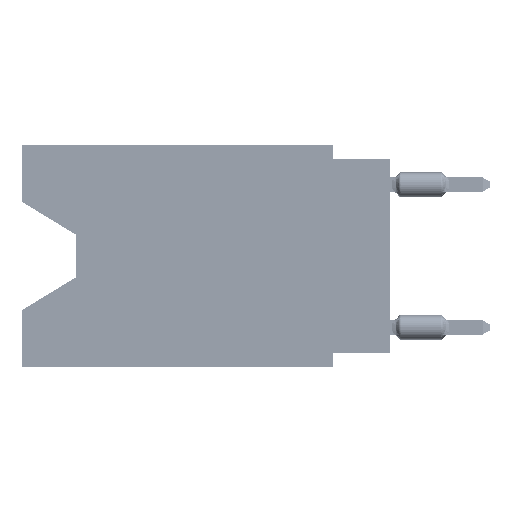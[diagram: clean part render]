
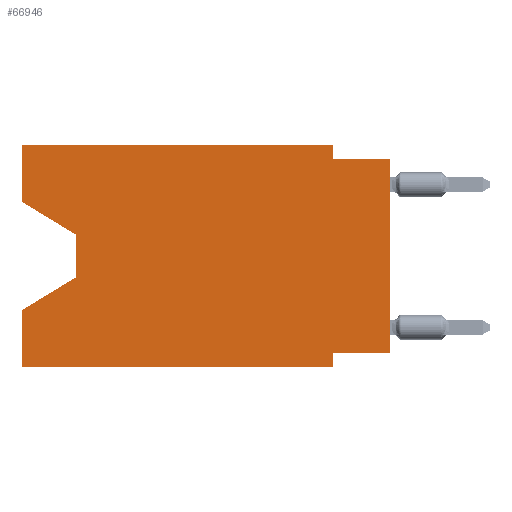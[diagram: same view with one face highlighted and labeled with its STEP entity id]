
A CAD part, left-side view. The second image highlights one B-rep face of the part: STEP entity #66946.
In plain terms, the highlighted planar face has unit normal (-1, 0, 0).
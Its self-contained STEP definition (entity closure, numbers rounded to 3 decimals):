
#549 = EDGE_CURVE ( 'NONE', #31729, #74322, #68696, .T. ) ;
#580 = DIRECTION ( 'NONE',  ( 0., 0., -1. ) ) ;
#655 = ORIENTED_EDGE ( 'NONE', *, *, #60571, .T. ) ;
#4515 = LINE ( 'NONE', #27219, #60084 ) ;
#5648 = EDGE_CURVE ( 'NONE', #44229, #64626, #75842, .T. ) ;
#5775 = CARTESIAN_POINT ( 'NONE',  ( 0., 13.97, -4.013 ) ) ;
#6532 = CARTESIAN_POINT ( 'NONE',  ( 0., 13.97, -4.013 ) ) ;
#7462 = DIRECTION ( 'NONE',  ( 0., -1., 0. ) ) ;
#8354 = CARTESIAN_POINT ( 'NONE',  ( 0., 0., -9.271 ) ) ;
#8669 = VERTEX_POINT ( 'NONE', #10261 ) ;
#9508 = LINE ( 'NONE', #32978, #18790 ) ;
#10261 = CARTESIAN_POINT ( 'NONE',  ( 0., 2.54, 0. ) ) ;
#12331 = VECTOR ( 'NONE', #63450, 1000. ) ;
#12679 = DIRECTION ( 'NONE',  ( 0., 0., -1. ) ) ;
#12710 = EDGE_CURVE ( 'NONE', #44229, #51005, #4515, .T. ) ;
#13248 = CARTESIAN_POINT ( 'NONE',  ( 0., 16.383, 0. ) ) ;
#13432 = CARTESIAN_POINT ( 'NONE',  ( 0., 16.383, -2.546 ) ) ;
#13996 = CARTESIAN_POINT ( 'NONE',  ( 0., 16.383, -9.906 ) ) ;
#15554 = CARTESIAN_POINT ( 'NONE',  ( 0., 16.383, -2.546 ) ) ;
#16294 = CARTESIAN_POINT ( 'NONE',  ( 0., 2.54, -9.906 ) ) ;
#16505 = DIRECTION ( 'NONE',  ( 0., -1., 0. ) ) ;
#18170 = ORIENTED_EDGE ( 'NONE', *, *, #21824, .T. ) ;
#18790 = VECTOR ( 'NONE', #27199, 1000. ) ;
#19012 = LINE ( 'NONE', #13248, #61201 ) ;
#19755 = LINE ( 'NONE', #13996, #71863 ) ;
#20933 = LINE ( 'NONE', #15554, #60937 ) ;
#21181 = EDGE_CURVE ( 'NONE', #67855, #69579, #70441, .T. ) ;
#21824 = EDGE_CURVE ( 'NONE', #45249, #54320, #19755, .T. ) ;
#24412 = CARTESIAN_POINT ( 'NONE',  ( 0., 16.383, 0. ) ) ;
#24763 = EDGE_CURVE ( 'NONE', #31729, #67855, #20933, .T. ) ;
#24780 = DIRECTION ( 'NONE',  ( 1., 0., 0. ) ) ;
#26344 = VECTOR ( 'NONE', #75595, 1000. ) ;
#27199 = DIRECTION ( 'NONE',  ( 0., 0., -1. ) ) ;
#27219 = CARTESIAN_POINT ( 'NONE',  ( 0., 0., -9.271 ) ) ;
#27464 = LINE ( 'NONE', #16294, #49008 ) ;
#27973 = DIRECTION ( 'NONE',  ( 0., 1., 0. ) ) ;
#30022 = DIRECTION ( 'NONE',  ( 0., 0., 1. ) ) ;
#31729 = VERTEX_POINT ( 'NONE', #13432 ) ;
#32461 = DIRECTION ( 'NONE',  ( 0., -1., 0. ) ) ;
#32978 = CARTESIAN_POINT ( 'NONE',  ( 0., 2.54, 0. ) ) ;
#34041 = CARTESIAN_POINT ( 'NONE',  ( 0., 16.383, 0. ) ) ;
#34280 = CARTESIAN_POINT ( 'NONE',  ( 0., 16.383, -7.36 ) ) ;
#36016 = ORIENTED_EDGE ( 'NONE', *, *, #68844, .F. ) ;
#36351 = CARTESIAN_POINT ( 'NONE',  ( 0., 16.383, 0. ) ) ;
#37364 = VECTOR ( 'NONE', #12679, 1000. ) ;
#37434 = VECTOR ( 'NONE', #16505, 1000. ) ;
#38621 = ORIENTED_EDGE ( 'NONE', *, *, #49227, .F. ) ;
#40558 = EDGE_CURVE ( 'NONE', #51005, #54320, #27464, .T. ) ;
#40971 = VERTEX_POINT ( 'NONE', #71398 ) ;
#42014 = CARTESIAN_POINT ( 'NONE',  ( 0., 0., -0.635 ) ) ;
#42133 = DIRECTION ( 'NONE',  ( 0., 0., 1. ) ) ;
#43893 = VECTOR ( 'NONE', #30022, 1000. ) ;
#44097 = ORIENTED_EDGE ( 'NONE', *, *, #56351, .F. ) ;
#44229 = VERTEX_POINT ( 'NONE', #8354 ) ;
#44473 = EDGE_CURVE ( 'NONE', #8669, #40971, #9508, .T. ) ;
#45249 = VERTEX_POINT ( 'NONE', #55296 ) ;
#45947 = DIRECTION ( 'NONE',  ( 0., 0., -1. ) ) ;
#46115 = VECTOR ( 'NONE', #42133, 1000. ) ;
#46597 = CARTESIAN_POINT ( 'NONE',  ( 0., 0., 0. ) ) ;
#48412 = VERTEX_POINT ( 'NONE', #34280 ) ;
#49008 = VECTOR ( 'NONE', #45947, 1000. ) ;
#49227 = EDGE_CURVE ( 'NONE', #74322, #8669, #19012, .T. ) ;
#49773 = CARTESIAN_POINT ( 'NONE',  ( 0., 16.383, 0. ) ) ;
#51005 = VERTEX_POINT ( 'NONE', #74105 ) ;
#51934 = CARTESIAN_POINT ( 'NONE',  ( 0., 0., -0.635 ) ) ;
#54061 = PLANE ( 'NONE',  #75445 ) ;
#54320 = VERTEX_POINT ( 'NONE', #56842 ) ;
#55296 = CARTESIAN_POINT ( 'NONE',  ( 0., 16.383, -9.906 ) ) ;
#56351 = EDGE_CURVE ( 'NONE', #45249, #48412, #70998, .T. ) ;
#56842 = CARTESIAN_POINT ( 'NONE',  ( 0., 2.54, -9.906 ) ) ;
#57715 = LINE ( 'NONE', #51934, #37434 ) ;
#59838 = FACE_OUTER_BOUND ( 'NONE', #73052, .T. ) ;
#60084 = VECTOR ( 'NONE', #27973, 1000. ) ;
#60571 = EDGE_CURVE ( 'NONE', #69579, #48412, #69600, .T. ) ;
#60937 = VECTOR ( 'NONE', #67906, 1000. ) ;
#61201 = VECTOR ( 'NONE', #7462, 1000. ) ;
#62742 = ORIENTED_EDGE ( 'NONE', *, *, #24763, .T. ) ;
#62860 = ORIENTED_EDGE ( 'NONE', *, *, #12710, .F. ) ;
#63068 = CARTESIAN_POINT ( 'NONE',  ( 0., 13.97, -5.893 ) ) ;
#63128 = ORIENTED_EDGE ( 'NONE', *, *, #44473, .F. ) ;
#63450 = DIRECTION ( 'NONE',  ( 0., 0.855, -0.519 ) ) ;
#64626 = VERTEX_POINT ( 'NONE', #42014 ) ;
#66946 = ADVANCED_FACE ( 'NONE', ( #59838 ), #54061, .F. ) ;
#67855 = VERTEX_POINT ( 'NONE', #5775 ) ;
#67906 = DIRECTION ( 'NONE',  ( 0., -0.855, -0.519 ) ) ;
#68696 = LINE ( 'NONE', #34041, #26344 ) ;
#68844 = EDGE_CURVE ( 'NONE', #40971, #64626, #57715, .T. ) ;
#69579 = VERTEX_POINT ( 'NONE', #75506 ) ;
#69600 = LINE ( 'NONE', #63068, #12331 ) ;
#70441 = LINE ( 'NONE', #6532, #37364 ) ;
#70448 = ORIENTED_EDGE ( 'NONE', *, *, #549, .F. ) ;
#70998 = LINE ( 'NONE', #36351, #46115 ) ;
#71165 = ORIENTED_EDGE ( 'NONE', *, *, #40558, .F. ) ;
#71398 = CARTESIAN_POINT ( 'NONE',  ( 0., 2.54, -0.635 ) ) ;
#71863 = VECTOR ( 'NONE', #32461, 1000. ) ;
#73052 = EDGE_LOOP ( 'NONE', ( #62742, #73744, #655, #44097, #18170, #71165, #62860, #75037, #36016, #63128, #38621, #70448 ) ) ;
#73744 = ORIENTED_EDGE ( 'NONE', *, *, #21181, .T. ) ;
#74105 = CARTESIAN_POINT ( 'NONE',  ( 0., 2.54, -9.271 ) ) ;
#74322 = VERTEX_POINT ( 'NONE', #49773 ) ;
#75037 = ORIENTED_EDGE ( 'NONE', *, *, #5648, .T. ) ;
#75445 = AXIS2_PLACEMENT_3D ( 'NONE', #24412, #24780, #580 ) ;
#75506 = CARTESIAN_POINT ( 'NONE',  ( 0., 13.97, -5.893 ) ) ;
#75595 = DIRECTION ( 'NONE',  ( 0., 0., 1. ) ) ;
#75842 = LINE ( 'NONE', #46597, #43893 ) ;
